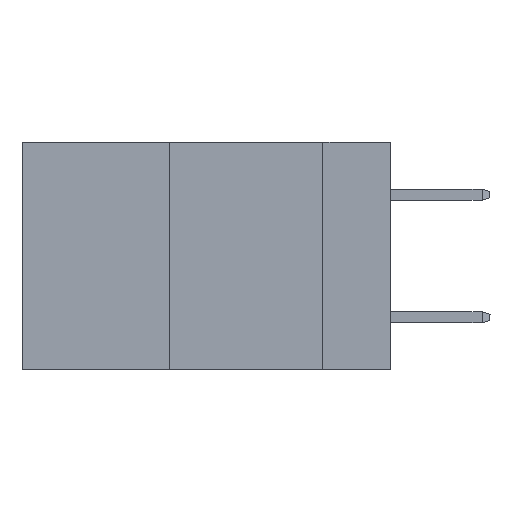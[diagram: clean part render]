
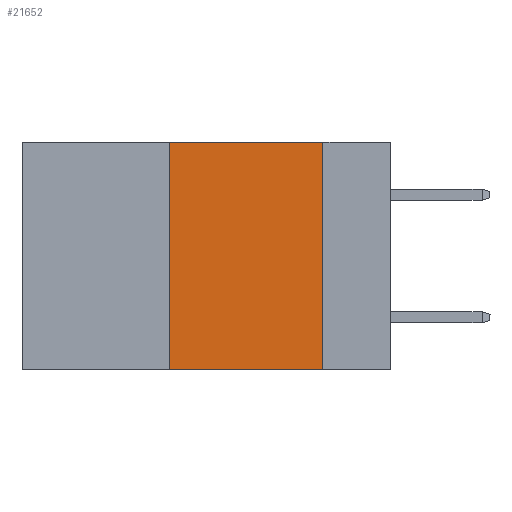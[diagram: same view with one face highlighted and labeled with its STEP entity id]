
A CAD part, left-side view. The second image highlights one B-rep face of the part: STEP entity #21652.
In plain terms, the highlighted planar face has unit normal (-1, 0, 0).
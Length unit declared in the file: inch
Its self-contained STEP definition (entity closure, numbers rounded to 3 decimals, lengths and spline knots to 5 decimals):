
#1662 = DIRECTION ( 'NONE',  ( 1., 0., 0. ) ) ;
#2099 = VECTOR ( 'NONE', #20077, 39.37008 ) ;
#2972 = VECTOR ( 'NONE', #19793, 39.37008 ) ;
#3064 = EDGE_CURVE ( 'NONE', #13696, #23062, #26792, .T. ) ;
#4170 = VECTOR ( 'NONE', #43053, 39.37008 ) ;
#5725 = CARTESIAN_POINT ( 'NONE',  ( 0., 0.36, -0.37 ) ) ;
#5962 = EDGE_CURVE ( 'NONE', #35093, #10065, #21713, .T. ) ;
#6395 = AXIS2_PLACEMENT_3D ( 'NONE', #11630, #1662, #15641 ) ;
#6421 = CARTESIAN_POINT ( 'NONE',  ( 0., 0.6, 0. ) ) ;
#6994 = FACE_OUTER_BOUND ( 'NONE', #7361, .T. ) ;
#7361 = EDGE_LOOP ( 'NONE', ( #10373, #40558, #40775, #31078 ) ) ;
#7631 = CARTESIAN_POINT ( 'NONE',  ( 0., 0.11, 0. ) ) ;
#10065 = VERTEX_POINT ( 'NONE', #42151 ) ;
#10373 = ORIENTED_EDGE ( 'NONE', *, *, #37555, .F. ) ;
#11630 = CARTESIAN_POINT ( 'NONE',  ( 0., 0.6, 0. ) ) ;
#12055 = VECTOR ( 'NONE', #24580, 39.37008 ) ;
#13276 = CARTESIAN_POINT ( 'NONE',  ( 0., 0.6, -0.37 ) ) ;
#13696 = VERTEX_POINT ( 'NONE', #32879 ) ;
#15641 = DIRECTION ( 'NONE',  ( 0., 0., -1. ) ) ;
#16163 = LINE ( 'NONE', #23205, #2972 ) ;
#17858 = CARTESIAN_POINT ( 'NONE',  ( 0., 0.11, 0. ) ) ;
#18586 = PLANE ( 'NONE',  #6395 ) ;
#19793 = DIRECTION ( 'NONE',  ( 0., 0., 1. ) ) ;
#19882 = EDGE_CURVE ( 'NONE', #35093, #13696, #16163, .T. ) ;
#20077 = DIRECTION ( 'NONE',  ( 0., -1., 0. ) ) ;
#21052 = LINE ( 'NONE', #7631, #12055 ) ;
#21652 = ADVANCED_FACE ( 'NONE', ( #6994 ), #18586, .F. ) ;
#21713 = LINE ( 'NONE', #13276, #2099 ) ;
#23062 = VERTEX_POINT ( 'NONE', #17858 ) ;
#23205 = CARTESIAN_POINT ( 'NONE',  ( 0., 0.36, 0. ) ) ;
#24580 = DIRECTION ( 'NONE',  ( 0., 0., -1. ) ) ;
#26792 = LINE ( 'NONE', #6421, #4170 ) ;
#31078 = ORIENTED_EDGE ( 'NONE', *, *, #5962, .T. ) ;
#32879 = CARTESIAN_POINT ( 'NONE',  ( 0., 0.36, 0. ) ) ;
#35093 = VERTEX_POINT ( 'NONE', #5725 ) ;
#37555 = EDGE_CURVE ( 'NONE', #23062, #10065, #21052, .T. ) ;
#40558 = ORIENTED_EDGE ( 'NONE', *, *, #3064, .F. ) ;
#40775 = ORIENTED_EDGE ( 'NONE', *, *, #19882, .F. ) ;
#42151 = CARTESIAN_POINT ( 'NONE',  ( 0., 0.11, -0.37 ) ) ;
#43053 = DIRECTION ( 'NONE',  ( 0., -1., 0. ) ) ;
